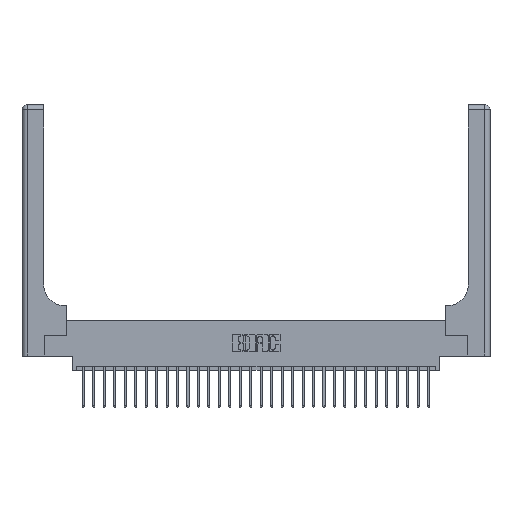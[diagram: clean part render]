
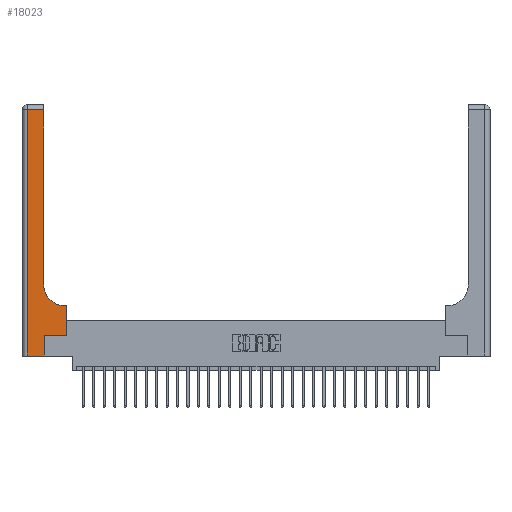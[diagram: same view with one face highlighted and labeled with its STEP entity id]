
A CAD part, top view. The second image highlights one B-rep face of the part: STEP entity #18023.
In plain terms, the highlighted planar face has unit normal (0, 0, 1).
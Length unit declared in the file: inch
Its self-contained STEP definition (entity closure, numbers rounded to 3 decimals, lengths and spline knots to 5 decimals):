
#277 = VECTOR ( 'NONE', #16935, 39.37008 ) ;
#810 = CARTESIAN_POINT ( 'NONE',  ( 0., 3., 0.37 ) ) ;
#822 = LINE ( 'NONE', #16084, #23757 ) ;
#936 = VERTEX_POINT ( 'NONE', #1592 ) ;
#992 = LINE ( 'NONE', #1351, #277 ) ;
#1308 = EDGE_CURVE ( 'NONE', #25340, #19979, #822, .T. ) ;
#1351 = CARTESIAN_POINT ( 'NONE',  ( 0., 2.94, 0.37 ) ) ;
#1592 = CARTESIAN_POINT ( 'NONE',  ( 0.06, 0., 0.37 ) ) ;
#2246 = VERTEX_POINT ( 'NONE', #6369 ) ;
#2888 = CARTESIAN_POINT ( 'NONE',  ( 0.51, 0.6, 0.37 ) ) ;
#3478 = VERTEX_POINT ( 'NONE', #21438 ) ;
#4284 = DIRECTION ( 'NONE',  ( 0., 0., -1. ) ) ;
#4842 = FACE_OUTER_BOUND ( 'NONE', #15224, .T. ) ;
#5345 = VERTEX_POINT ( 'NONE', #24738 ) ;
#5736 = LINE ( 'NONE', #15349, #28420 ) ;
#6264 = ORIENTED_EDGE ( 'NONE', *, *, #8930, .T. ) ;
#6365 = ORIENTED_EDGE ( 'NONE', *, *, #17450, .T. ) ;
#6369 = CARTESIAN_POINT ( 'NONE',  ( 0.06, 2.94, 0.37 ) ) ;
#6676 = VECTOR ( 'NONE', #26436, 39.37008 ) ;
#6760 = LINE ( 'NONE', #16970, #23694 ) ;
#6791 = ORIENTED_EDGE ( 'NONE', *, *, #22138, .T. ) ;
#8930 = EDGE_CURVE ( 'NONE', #28606, #24708, #14307, .T. ) ;
#9272 = EDGE_CURVE ( 'NONE', #24708, #27196, #19149, .T. ) ;
#9519 = DIRECTION ( 'NONE',  ( 0., 1., 0. ) ) ;
#9992 = EDGE_CURVE ( 'NONE', #27196, #2246, #992, .T. ) ;
#10223 = CARTESIAN_POINT ( 'NONE',  ( 0.265, 0.25, 0.37 ) ) ;
#10371 = AXIS2_PLACEMENT_3D ( 'NONE', #810, #12048, #27393 ) ;
#11291 = CARTESIAN_POINT ( 'NONE',  ( 0.26, 2.94, 0.37 ) ) ;
#11470 = VECTOR ( 'NONE', #23199, 39.37008 ) ;
#11960 = PLANE ( 'NONE',  #10371 ) ;
#12048 = DIRECTION ( 'NONE',  ( 0., 0., -1. ) ) ;
#12573 = VECTOR ( 'NONE', #14543, 39.37008 ) ;
#14307 = CIRCLE ( 'NONE', #20369, 0.25 ) ;
#14543 = DIRECTION ( 'NONE',  ( 0., 1., 0. ) ) ;
#14799 = EDGE_CURVE ( 'NONE', #3478, #5345, #5736, .T. ) ;
#14938 = CARTESIAN_POINT ( 'NONE',  ( 0.265, 0., 0.37 ) ) ;
#14968 = CARTESIAN_POINT ( 'NONE',  ( 0.26, 0.85, 0.37 ) ) ;
#15224 = EDGE_LOOP ( 'NONE', ( #28506, #27351, #26648, #17768, #21165, #6791, #19296, #6365, #6264 ) ) ;
#15349 = CARTESIAN_POINT ( 'NONE',  ( 0.528, 0.25, 0.37 ) ) ;
#16084 = CARTESIAN_POINT ( 'NONE',  ( 0.265, 0., 0.37 ) ) ;
#16935 = DIRECTION ( 'NONE',  ( -1., 0., 0. ) ) ;
#16970 = CARTESIAN_POINT ( 'NONE',  ( 0.265, 0.25, 0.37 ) ) ;
#17450 = EDGE_CURVE ( 'NONE', #5345, #28606, #23221, .T. ) ;
#17565 = CARTESIAN_POINT ( 'NONE',  ( 0.51, 0.85, 0.37 ) ) ;
#17741 = CARTESIAN_POINT ( 'NONE',  ( 0.06, 3., 0.37 ) ) ;
#17768 = ORIENTED_EDGE ( 'NONE', *, *, #23330, .T. ) ;
#18023 = ADVANCED_FACE ( 'NONE', ( #4842 ), #11960, .F. ) ;
#18126 = VECTOR ( 'NONE', #18743, 39.37008 ) ;
#18456 = LINE ( 'NONE', #17741, #6676 ) ;
#18743 = DIRECTION ( 'NONE',  ( 1., 0., 0. ) ) ;
#19149 = LINE ( 'NONE', #21153, #12573 ) ;
#19296 = ORIENTED_EDGE ( 'NONE', *, *, #14799, .T. ) ;
#19805 = DIRECTION ( 'NONE',  ( 1., 0., 0. ) ) ;
#19979 = VERTEX_POINT ( 'NONE', #10223 ) ;
#20369 = AXIS2_PLACEMENT_3D ( 'NONE', #17565, #4284, #19805 ) ;
#21004 = CARTESIAN_POINT ( 'NONE',  ( 0.26, 0.6, 0.37 ) ) ;
#21153 = CARTESIAN_POINT ( 'NONE',  ( 0.26, 3., 0.37 ) ) ;
#21165 = ORIENTED_EDGE ( 'NONE', *, *, #1308, .T. ) ;
#21438 = CARTESIAN_POINT ( 'NONE',  ( 0.528, 0.25, 0.37 ) ) ;
#22028 = DIRECTION ( 'NONE',  ( 0., 1., 0. ) ) ;
#22138 = EDGE_CURVE ( 'NONE', #19979, #3478, #6760, .T. ) ;
#23199 = DIRECTION ( 'NONE',  ( -1., 0., 0. ) ) ;
#23221 = LINE ( 'NONE', #21004, #11470 ) ;
#23301 = LINE ( 'NONE', #23352, #18126 ) ;
#23330 = EDGE_CURVE ( 'NONE', #936, #25340, #23301, .T. ) ;
#23352 = CARTESIAN_POINT ( 'NONE',  ( 0., 0., 0.37 ) ) ;
#23523 = EDGE_CURVE ( 'NONE', #2246, #936, #18456, .T. ) ;
#23624 = DIRECTION ( 'NONE',  ( 1., 0., 0. ) ) ;
#23694 = VECTOR ( 'NONE', #23624, 39.37008 ) ;
#23757 = VECTOR ( 'NONE', #9519, 39.37008 ) ;
#24708 = VERTEX_POINT ( 'NONE', #14968 ) ;
#24738 = CARTESIAN_POINT ( 'NONE',  ( 0.528, 0.6, 0.37 ) ) ;
#25340 = VERTEX_POINT ( 'NONE', #14938 ) ;
#26436 = DIRECTION ( 'NONE',  ( 0., -1., 0. ) ) ;
#26648 = ORIENTED_EDGE ( 'NONE', *, *, #23523, .T. ) ;
#27196 = VERTEX_POINT ( 'NONE', #11291 ) ;
#27351 = ORIENTED_EDGE ( 'NONE', *, *, #9992, .T. ) ;
#27393 = DIRECTION ( 'NONE',  ( -1., 0., 0. ) ) ;
#28420 = VECTOR ( 'NONE', #22028, 39.37008 ) ;
#28506 = ORIENTED_EDGE ( 'NONE', *, *, #9272, .T. ) ;
#28606 = VERTEX_POINT ( 'NONE', #2888 ) ;
